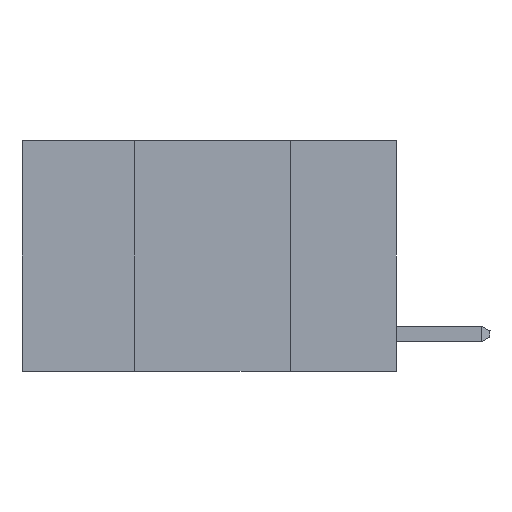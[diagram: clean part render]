
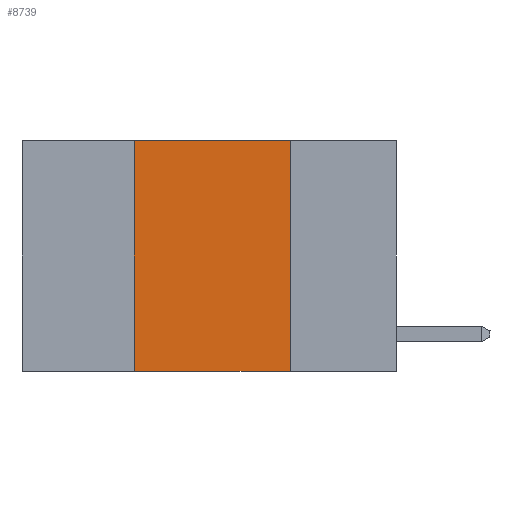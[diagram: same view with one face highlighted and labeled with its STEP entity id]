
A CAD part, left-side view. The second image highlights one B-rep face of the part: STEP entity #8739.
In plain terms, the highlighted planar face has unit normal (-1, 0, 0).
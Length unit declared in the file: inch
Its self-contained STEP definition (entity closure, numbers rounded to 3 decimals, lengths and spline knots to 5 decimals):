
#87 = VERTEX_POINT ( 'NONE', #3860 ) ;
#590 = PLANE ( 'NONE',  #10925 ) ;
#945 = EDGE_LOOP ( 'NONE', ( #4275, #6599, #6813, #10655 ) ) ;
#1212 = LINE ( 'NONE', #9573, #9487 ) ;
#2104 = DIRECTION ( 'NONE',  ( 0., -1., 0. ) ) ;
#3121 = DIRECTION ( 'NONE',  ( 0., -1., 0. ) ) ;
#3280 = CARTESIAN_POINT ( 'NONE',  ( 0., 0.42, 0. ) ) ;
#3454 = VERTEX_POINT ( 'NONE', #7880 ) ;
#3860 = CARTESIAN_POINT ( 'NONE',  ( 0., 0.42, -0.37 ) ) ;
#3865 = DIRECTION ( 'NONE',  ( 1., 0., 0. ) ) ;
#4275 = ORIENTED_EDGE ( 'NONE', *, *, #5263, .F. ) ;
#4580 = DIRECTION ( 'NONE',  ( 0., 0., -1. ) ) ;
#5263 = EDGE_CURVE ( 'NONE', #3454, #8335, #7008, .T. ) ;
#5325 = CARTESIAN_POINT ( 'NONE',  ( 0., 0.42, 0. ) ) ;
#6394 = DIRECTION ( 'NONE',  ( 0., 0., 1. ) ) ;
#6430 = VECTOR ( 'NONE', #6394, 39.37008 ) ;
#6599 = ORIENTED_EDGE ( 'NONE', *, *, #12027, .F. ) ;
#6650 = VECTOR ( 'NONE', #4580, 39.37008 ) ;
#6774 = LINE ( 'NONE', #5325, #6430 ) ;
#6813 = ORIENTED_EDGE ( 'NONE', *, *, #9831, .F. ) ;
#7008 = LINE ( 'NONE', #10977, #6650 ) ;
#7246 = VERTEX_POINT ( 'NONE', #3280 ) ;
#7526 = CARTESIAN_POINT ( 'NONE',  ( 0., 0.6, 0. ) ) ;
#7552 = VECTOR ( 'NONE', #2104, 39.37008 ) ;
#7647 = EDGE_CURVE ( 'NONE', #87, #8335, #1212, .T. ) ;
#7880 = CARTESIAN_POINT ( 'NONE',  ( 0., 0.17, 0. ) ) ;
#8335 = VERTEX_POINT ( 'NONE', #13762 ) ;
#8739 = ADVANCED_FACE ( 'NONE', ( #9478 ), #590, .F. ) ;
#9478 = FACE_OUTER_BOUND ( 'NONE', #945, .T. ) ;
#9487 = VECTOR ( 'NONE', #3121, 39.37008 ) ;
#9573 = CARTESIAN_POINT ( 'NONE',  ( 0., 0.6, -0.37 ) ) ;
#9831 = EDGE_CURVE ( 'NONE', #87, #7246, #6774, .T. ) ;
#10294 = CARTESIAN_POINT ( 'NONE',  ( 0., 0.6, 0. ) ) ;
#10364 = LINE ( 'NONE', #7526, #7552 ) ;
#10655 = ORIENTED_EDGE ( 'NONE', *, *, #7647, .T. ) ;
#10925 = AXIS2_PLACEMENT_3D ( 'NONE', #10294, #3865, #11333 ) ;
#10977 = CARTESIAN_POINT ( 'NONE',  ( 0., 0.17, 0. ) ) ;
#11333 = DIRECTION ( 'NONE',  ( 0., 0., -1. ) ) ;
#12027 = EDGE_CURVE ( 'NONE', #7246, #3454, #10364, .T. ) ;
#13762 = CARTESIAN_POINT ( 'NONE',  ( 0., 0.17, -0.37 ) ) ;
